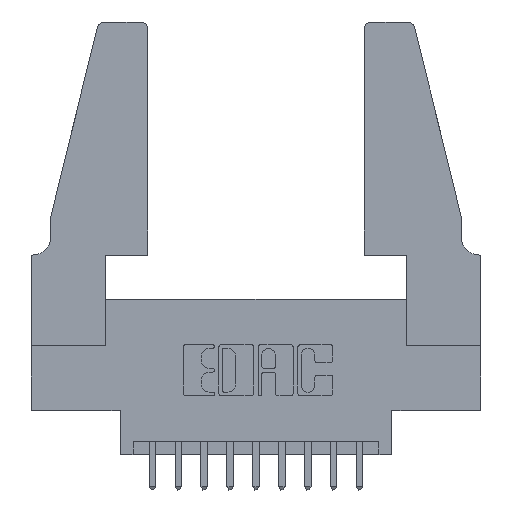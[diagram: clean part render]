
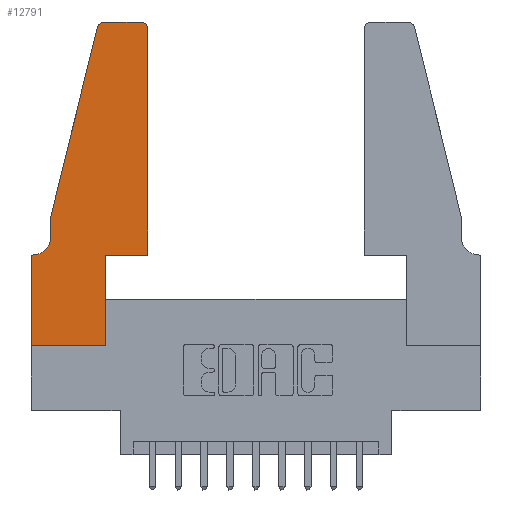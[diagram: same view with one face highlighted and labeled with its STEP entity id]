
A CAD part, top view. The second image highlights one B-rep face of the part: STEP entity #12791.
In plain terms, the highlighted planar face has unit normal (0, 0, 1).
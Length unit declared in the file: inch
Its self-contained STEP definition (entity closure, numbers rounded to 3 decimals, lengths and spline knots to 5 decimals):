
#176 = CIRCLE ( 'NONE', #6830, 0.07 ) ;
#186 = VERTEX_POINT ( 'NONE', #7890 ) ;
#253 = DIRECTION ( 'NONE',  ( 1., 0., 0. ) ) ;
#257 = VERTEX_POINT ( 'NONE', #10725 ) ;
#491 = LINE ( 'NONE', #3988, #3146 ) ;
#522 = EDGE_CURVE ( 'NONE', #9711, #9621, #1062, .T. ) ;
#591 = DIRECTION ( 'NONE',  ( 1., 0., 0. ) ) ;
#620 = DIRECTION ( 'NONE',  ( 1., 0., 0. ) ) ;
#864 = CARTESIAN_POINT ( 'NONE',  ( 0.2865, 0.35, 0.37 ) ) ;
#1062 = LINE ( 'NONE', #9551, #4030 ) ;
#1149 = CARTESIAN_POINT ( 'NONE',  ( 0.4205, 1.25, 0.37 ) ) ;
#1159 = EDGE_CURVE ( 'NONE', #257, #10996, #8658, .T. ) ;
#1225 = CARTESIAN_POINT ( 'NONE',  ( 0.4205, 1.22, 0.37 ) ) ;
#1896 = VECTOR ( 'NONE', #11712, 39.37008 ) ;
#2116 = VERTEX_POINT ( 'NONE', #10011 ) ;
#2119 = CARTESIAN_POINT ( 'NONE',  ( 0.0755, 0.5, 0.37 ) ) ;
#2240 = LINE ( 'NONE', #2119, #1896 ) ;
#2279 = VECTOR ( 'NONE', #8033, 39.37008 ) ;
#2370 = DIRECTION ( 'NONE',  ( 1., 0., 0. ) ) ;
#2493 = DIRECTION ( 'NONE',  ( 0., 0., 1. ) ) ;
#2527 = AXIS2_PLACEMENT_3D ( 'NONE', #1225, #8793, #2370 ) ;
#3146 = VECTOR ( 'NONE', #620, 39.37008 ) ;
#3170 = EDGE_CURVE ( 'NONE', #3560, #9711, #4441, .T. ) ;
#3414 = ORIENTED_EDGE ( 'NONE', *, *, #3170, .T. ) ;
#3560 = VERTEX_POINT ( 'NONE', #10916 ) ;
#3634 = EDGE_CURVE ( 'NONE', #12255, #257, #11873, .T. ) ;
#3756 = ORIENTED_EDGE ( 'NONE', *, *, #11967, .T. ) ;
#3959 = LINE ( 'NONE', #13382, #6427 ) ;
#3988 = CARTESIAN_POINT ( 'NONE',  ( 0., 0., 0.37 ) ) ;
#4030 = VECTOR ( 'NONE', #9525, 39.37008 ) ;
#4441 = LINE ( 'NONE', #6738, #6929 ) ;
#4618 = CARTESIAN_POINT ( 'NONE',  ( 0., 0.35, 0.37 ) ) ;
#4673 = EDGE_CURVE ( 'NONE', #4851, #12255, #4752, .T. ) ;
#4752 = LINE ( 'NONE', #11623, #13768 ) ;
#4792 = DIRECTION ( 'NONE',  ( 0., 0., -1. ) ) ;
#4850 = CIRCLE ( 'NONE', #2527, 0.03 ) ;
#4851 = VERTEX_POINT ( 'NONE', #1149 ) ;
#5231 = ORIENTED_EDGE ( 'NONE', *, *, #1159, .T. ) ;
#5269 = DIRECTION ( 'NONE',  ( -1., 0., 0. ) ) ;
#5383 = VERTEX_POINT ( 'NONE', #8613 ) ;
#5476 = EDGE_CURVE ( 'NONE', #5383, #4851, #4850, .T. ) ;
#5562 = LINE ( 'NONE', #8196, #10888 ) ;
#5635 = EDGE_CURVE ( 'NONE', #2116, #3560, #176, .T. ) ;
#6427 = VECTOR ( 'NONE', #8211, 39.37008 ) ;
#6499 = VERTEX_POINT ( 'NONE', #12938 ) ;
#6579 = FACE_OUTER_BOUND ( 'NONE', #13433, .T. ) ;
#6618 = DIRECTION ( 'NONE',  ( 0., 1., 0. ) ) ;
#6738 = CARTESIAN_POINT ( 'NONE',  ( 0.0755, 0.35, 0.37 ) ) ;
#6784 = DIRECTION ( 'NONE',  ( 0., 0., 1. ) ) ;
#6830 = AXIS2_PLACEMENT_3D ( 'NONE', #11128, #4792, #12178 ) ;
#6926 = VERTEX_POINT ( 'NONE', #864 ) ;
#6929 = VECTOR ( 'NONE', #7071, 39.37008 ) ;
#7071 = DIRECTION ( 'NONE',  ( -1., 0., 0. ) ) ;
#7252 = ORIENTED_EDGE ( 'NONE', *, *, #13738, .T. ) ;
#7418 = ORIENTED_EDGE ( 'NONE', *, *, #4673, .T. ) ;
#7701 = EDGE_CURVE ( 'NONE', #10996, #2116, #2240, .T. ) ;
#7890 = CARTESIAN_POINT ( 'NONE',  ( 0.2865, 0., 0.37 ) ) ;
#7998 = CARTESIAN_POINT ( 'NONE',  ( 0.284, 1.25, 0.37 ) ) ;
#8033 = DIRECTION ( 'NONE',  ( -0.239, -0.971, 0. ) ) ;
#8196 = CARTESIAN_POINT ( 'NONE',  ( 0.4505, 0.35, 0.37 ) ) ;
#8211 = DIRECTION ( 'NONE',  ( 0., 1., 0. ) ) ;
#8471 = CARTESIAN_POINT ( 'NONE',  ( 0., 0., 0.37 ) ) ;
#8613 = CARTESIAN_POINT ( 'NONE',  ( 0.4505, 1.22, 0.37 ) ) ;
#8639 = CARTESIAN_POINT ( 'NONE',  ( 0., 0.35, 0.37 ) ) ;
#8658 = LINE ( 'NONE', #11985, #2279 ) ;
#8679 = EDGE_CURVE ( 'NONE', #6499, #5383, #3959, .T. ) ;
#8739 = CARTESIAN_POINT ( 'NONE',  ( 0.0755, 0.5, 0.37 ) ) ;
#8793 = DIRECTION ( 'NONE',  ( 0., 0., 1. ) ) ;
#8888 = PLANE ( 'NONE',  #13456 ) ;
#9068 = ORIENTED_EDGE ( 'NONE', *, *, #522, .T. ) ;
#9417 = EDGE_CURVE ( 'NONE', #6926, #6499, #5562, .T. ) ;
#9525 = DIRECTION ( 'NONE',  ( 0., -1., 0. ) ) ;
#9551 = CARTESIAN_POINT ( 'NONE',  ( 0., 0., 0.37 ) ) ;
#9621 = VERTEX_POINT ( 'NONE', #8471 ) ;
#9711 = VERTEX_POINT ( 'NONE', #8639 ) ;
#9940 = DIRECTION ( 'NONE',  ( 1., 0., 0. ) ) ;
#10011 = CARTESIAN_POINT ( 'NONE',  ( 0.0755, 0.42, 0.37 ) ) ;
#10551 = ORIENTED_EDGE ( 'NONE', *, *, #3634, .T. ) ;
#10725 = CARTESIAN_POINT ( 'NONE',  ( 0.25487, 1.22718, 0.37 ) ) ;
#10805 = AXIS2_PLACEMENT_3D ( 'NONE', #13065, #6784, #253 ) ;
#10876 = ORIENTED_EDGE ( 'NONE', *, *, #7701, .T. ) ;
#10888 = VECTOR ( 'NONE', #591, 39.37008 ) ;
#10916 = CARTESIAN_POINT ( 'NONE',  ( 0.0055, 0.35, 0.37 ) ) ;
#10996 = VERTEX_POINT ( 'NONE', #8739 ) ;
#11128 = CARTESIAN_POINT ( 'NONE',  ( 0.0055, 0.42, 0.37 ) ) ;
#11206 = ORIENTED_EDGE ( 'NONE', *, *, #5635, .T. ) ;
#11623 = CARTESIAN_POINT ( 'NONE',  ( 0.2605, 1.25, 0.37 ) ) ;
#11712 = DIRECTION ( 'NONE',  ( 0., -1., 0. ) ) ;
#11856 = VECTOR ( 'NONE', #6618, 39.37008 ) ;
#11873 = CIRCLE ( 'NONE', #10805, 0.03 ) ;
#11967 = EDGE_CURVE ( 'NONE', #9621, #186, #491, .T. ) ;
#11985 = CARTESIAN_POINT ( 'NONE',  ( 0.0755, 0.5, 0.37 ) ) ;
#12178 = DIRECTION ( 'NONE',  ( -1., 0., 0. ) ) ;
#12255 = VERTEX_POINT ( 'NONE', #7998 ) ;
#12791 = ADVANCED_FACE ( 'NONE', ( #6579 ), #8888, .T. ) ;
#12820 = ORIENTED_EDGE ( 'NONE', *, *, #9417, .T. ) ;
#12915 = CARTESIAN_POINT ( 'NONE',  ( 0.2865, 0.35, 0.37 ) ) ;
#12938 = CARTESIAN_POINT ( 'NONE',  ( 0.4505, 0.35, 0.37 ) ) ;
#13065 = CARTESIAN_POINT ( 'NONE',  ( 0.284, 1.22, 0.37 ) ) ;
#13130 = ORIENTED_EDGE ( 'NONE', *, *, #8679, .T. ) ;
#13382 = CARTESIAN_POINT ( 'NONE',  ( 0.4505, 0.35, 0.37 ) ) ;
#13433 = EDGE_LOOP ( 'NONE', ( #7418, #10551, #5231, #10876, #11206, #3414, #9068, #3756, #7252, #12820, #13130, #13450 ) ) ;
#13450 = ORIENTED_EDGE ( 'NONE', *, *, #5476, .T. ) ;
#13456 = AXIS2_PLACEMENT_3D ( 'NONE', #4618, #2493, #9940 ) ;
#13610 = LINE ( 'NONE', #12915, #11856 ) ;
#13738 = EDGE_CURVE ( 'NONE', #186, #6926, #13610, .T. ) ;
#13768 = VECTOR ( 'NONE', #5269, 39.37008 ) ;
